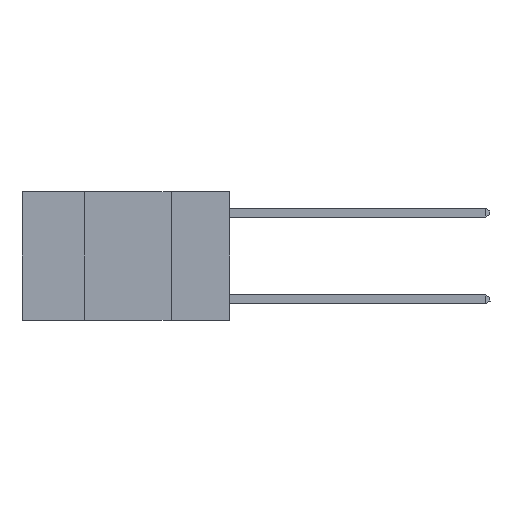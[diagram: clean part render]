
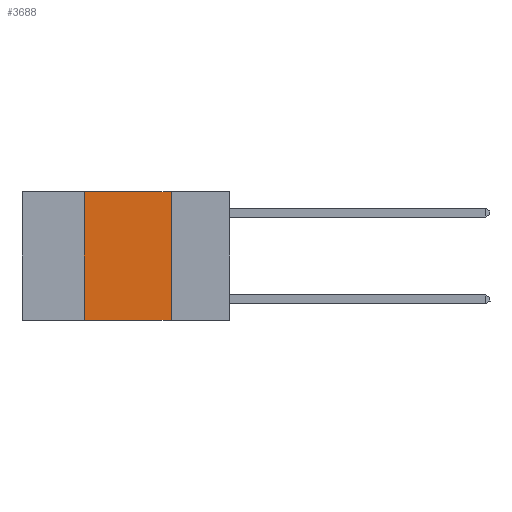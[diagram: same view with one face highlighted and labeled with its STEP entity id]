
A CAD part, left-side view. The second image highlights one B-rep face of the part: STEP entity #3688.
In plain terms, the highlighted planar face has unit normal (-1, 0, 0).
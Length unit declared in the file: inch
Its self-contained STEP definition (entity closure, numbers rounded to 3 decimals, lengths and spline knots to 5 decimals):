
#291 = DIRECTION ( 'NONE',  ( 0., 0., -1. ) ) ;
#298 = LINE ( 'NONE', #11892, #8342 ) ;
#1869 = CARTESIAN_POINT ( 'NONE',  ( 0., 0.42, -0.37 ) ) ;
#1945 = EDGE_CURVE ( 'NONE', #2152, #6141, #16478, .T. ) ;
#2152 = VERTEX_POINT ( 'NONE', #6191 ) ;
#2217 = CARTESIAN_POINT ( 'NONE',  ( 0., 0.6, 0. ) ) ;
#2575 = LINE ( 'NONE', #3385, #9885 ) ;
#2865 = CARTESIAN_POINT ( 'NONE',  ( 0., 0.17, 0. ) ) ;
#3385 = CARTESIAN_POINT ( 'NONE',  ( 0., 0.42, 0. ) ) ;
#3570 = DIRECTION ( 'NONE',  ( 1., 0., 0. ) ) ;
#3688 = ADVANCED_FACE ( 'NONE', ( #10728 ), #18775, .F. ) ;
#4282 = DIRECTION ( 'NONE',  ( 0., -1., 0. ) ) ;
#4337 = VECTOR ( 'NONE', #11486, 39.37008 ) ;
#6141 = VERTEX_POINT ( 'NONE', #7655 ) ;
#6191 = CARTESIAN_POINT ( 'NONE',  ( 0., 0.42, 0. ) ) ;
#7546 = CARTESIAN_POINT ( 'NONE',  ( 0., 0.17, -0.37 ) ) ;
#7573 = AXIS2_PLACEMENT_3D ( 'NONE', #17285, #3570, #291 ) ;
#7655 = CARTESIAN_POINT ( 'NONE',  ( 0., 0.17, 0. ) ) ;
#8342 = VECTOR ( 'NONE', #4282, 39.37008 ) ;
#9885 = VECTOR ( 'NONE', #17122, 39.37008 ) ;
#10728 = FACE_OUTER_BOUND ( 'NONE', #17149, .T. ) ;
#11477 = ORIENTED_EDGE ( 'NONE', *, *, #13749, .F. ) ;
#11486 = DIRECTION ( 'NONE',  ( 0., -1., 0. ) ) ;
#11892 = CARTESIAN_POINT ( 'NONE',  ( 0., 0.6, -0.37 ) ) ;
#11935 = ORIENTED_EDGE ( 'NONE', *, *, #13978, .F. ) ;
#12186 = DIRECTION ( 'NONE',  ( 0., 0., -1. ) ) ;
#12695 = EDGE_CURVE ( 'NONE', #14993, #16324, #298, .T. ) ;
#13749 = EDGE_CURVE ( 'NONE', #6141, #16324, #17700, .T. ) ;
#13978 = EDGE_CURVE ( 'NONE', #14993, #2152, #2575, .T. ) ;
#14993 = VERTEX_POINT ( 'NONE', #1869 ) ;
#15479 = ORIENTED_EDGE ( 'NONE', *, *, #1945, .F. ) ;
#16324 = VERTEX_POINT ( 'NONE', #7546 ) ;
#16478 = LINE ( 'NONE', #2217, #4337 ) ;
#17122 = DIRECTION ( 'NONE',  ( 0., 0., 1. ) ) ;
#17149 = EDGE_LOOP ( 'NONE', ( #11477, #15479, #11935, #19484 ) ) ;
#17220 = VECTOR ( 'NONE', #12186, 39.37008 ) ;
#17285 = CARTESIAN_POINT ( 'NONE',  ( 0., 0.6, 0. ) ) ;
#17700 = LINE ( 'NONE', #2865, #17220 ) ;
#18775 = PLANE ( 'NONE',  #7573 ) ;
#19484 = ORIENTED_EDGE ( 'NONE', *, *, #12695, .T. ) ;
